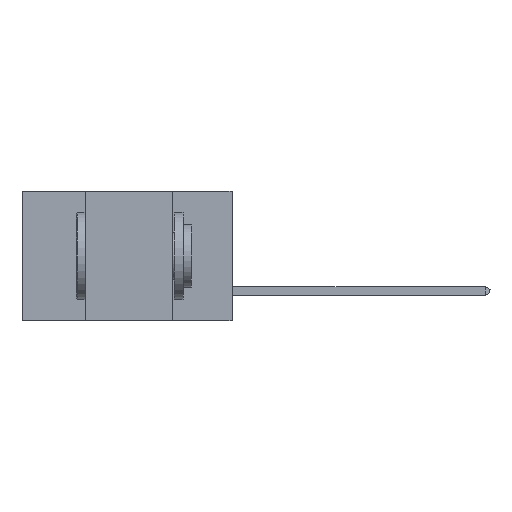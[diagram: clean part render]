
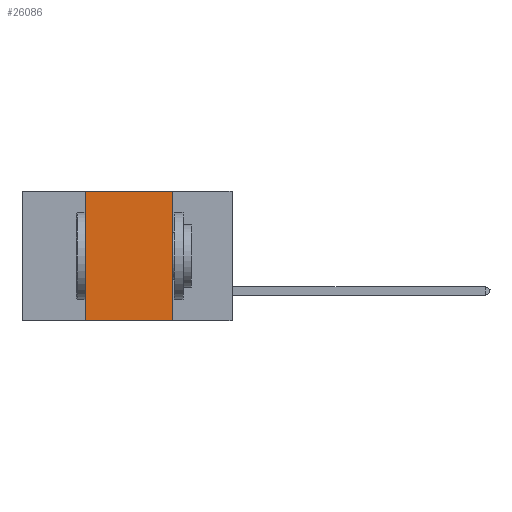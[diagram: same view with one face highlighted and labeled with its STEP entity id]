
A CAD part, left-side view. The second image highlights one B-rep face of the part: STEP entity #26086.
In plain terms, the highlighted planar face has unit normal (-1, 0, 0).
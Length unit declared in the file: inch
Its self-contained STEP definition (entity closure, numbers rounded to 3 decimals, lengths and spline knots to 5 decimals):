
#1275 = CARTESIAN_POINT ( 'NONE',  ( 0., 0.17, 0. ) ) ;
#1899 = DIRECTION ( 'NONE',  ( 0., 0., -1. ) ) ;
#2110 = CARTESIAN_POINT ( 'NONE',  ( 0., 0.17, 0. ) ) ;
#2683 = EDGE_CURVE ( 'NONE', #18915, #24756, #9497, .T. ) ;
#6135 = DIRECTION ( 'NONE',  ( 0., 0., -1. ) ) ;
#6784 = CARTESIAN_POINT ( 'NONE',  ( 0., 0.42, -0.37 ) ) ;
#7094 = CARTESIAN_POINT ( 'NONE',  ( 0., 0.42, 0. ) ) ;
#8282 = VERTEX_POINT ( 'NONE', #1275 ) ;
#8751 = VECTOR ( 'NONE', #16744, 39.37008 ) ;
#8838 = EDGE_CURVE ( 'NONE', #18915, #23476, #22687, .T. ) ;
#8875 = EDGE_CURVE ( 'NONE', #8282, #24756, #16362, .T. ) ;
#8924 = EDGE_LOOP ( 'NONE', ( #24344, #30256, #26364, #9804 ) ) ;
#9497 = LINE ( 'NONE', #27232, #26792 ) ;
#9804 = ORIENTED_EDGE ( 'NONE', *, *, #2683, .T. ) ;
#12380 = EDGE_CURVE ( 'NONE', #23476, #8282, #18707, .T. ) ;
#13610 = AXIS2_PLACEMENT_3D ( 'NONE', #25167, #25356, #1899 ) ;
#13787 = CARTESIAN_POINT ( 'NONE',  ( 0., 0.17, -0.37 ) ) ;
#15058 = VECTOR ( 'NONE', #28844, 39.37008 ) ;
#16362 = LINE ( 'NONE', #2110, #20096 ) ;
#16744 = DIRECTION ( 'NONE',  ( 0., 0., 1. ) ) ;
#17284 = CARTESIAN_POINT ( 'NONE',  ( 0., 0.6, 0. ) ) ;
#17494 = FACE_OUTER_BOUND ( 'NONE', #8924, .T. ) ;
#17867 = CARTESIAN_POINT ( 'NONE',  ( 0., 0.42, 0. ) ) ;
#18056 = PLANE ( 'NONE',  #13610 ) ;
#18707 = LINE ( 'NONE', #17284, #15058 ) ;
#18915 = VERTEX_POINT ( 'NONE', #6784 ) ;
#20096 = VECTOR ( 'NONE', #6135, 39.37008 ) ;
#22687 = LINE ( 'NONE', #7094, #8751 ) ;
#23476 = VERTEX_POINT ( 'NONE', #17867 ) ;
#24344 = ORIENTED_EDGE ( 'NONE', *, *, #8875, .F. ) ;
#24756 = VERTEX_POINT ( 'NONE', #13787 ) ;
#25167 = CARTESIAN_POINT ( 'NONE',  ( 0., 0.6, 0. ) ) ;
#25356 = DIRECTION ( 'NONE',  ( 1., 0., 0. ) ) ;
#26086 = ADVANCED_FACE ( 'NONE', ( #17494 ), #18056, .F. ) ;
#26364 = ORIENTED_EDGE ( 'NONE', *, *, #8838, .F. ) ;
#26792 = VECTOR ( 'NONE', #29297, 39.37008 ) ;
#27232 = CARTESIAN_POINT ( 'NONE',  ( 0., 0.6, -0.37 ) ) ;
#28844 = DIRECTION ( 'NONE',  ( 0., -1., 0. ) ) ;
#29297 = DIRECTION ( 'NONE',  ( 0., -1., 0. ) ) ;
#30256 = ORIENTED_EDGE ( 'NONE', *, *, #12380, .F. ) ;
